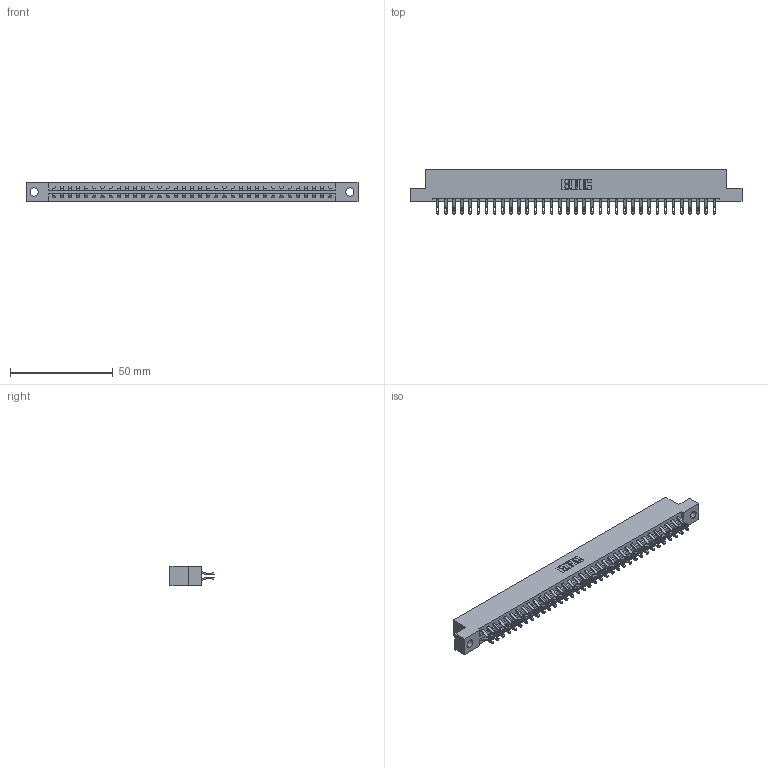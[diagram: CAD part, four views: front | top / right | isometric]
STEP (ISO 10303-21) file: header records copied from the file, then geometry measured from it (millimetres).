
FILE_DESCRIPTION (( 'STEP AP203' ), '1' );
FILE_NAME ('387-070-555-204.STEP', '2019-10-21T22:49:55', ( '' ), ( '' ), 'SwSTEP 2.0', 'SolidWorks 2016', '' );
FILE_SCHEMA (( 'CONFIG_CONTROL_DESIGN' ));
Length unit declared in the file: inch
Products named in the file (3): 345-292-001_555 Tail; 387-070-555-204; 337 Part_Flush Mounting Lugs - 0.156 Dia-TH
Assembly tree (71 placements, depth 2):
  387-070-555-204
    337 Part_Flush Mounting Lugs - 0.156 Dia-TH
    345-292-001_555 Tail  x70
Bounding box: 161.7 x 21.47 x 9.4 mm (x, y, z)
Volume: 17062.9 mm3; surface area: 19784.1 mm2
Topology: 71 solids, 71 shells, 4314 faces, 13541 edges, 9026 vertices
Faces by surface type: plane 2590, cylinder 1724
Entity records: 28371 total; most frequent: CARTESIAN_POINT 4820, ORIENTED_EDGE 4726, DIRECTION 4083, EDGE_CURVE 2363, VECTOR 2215, LINE 2215, VERTEX_POINT 1574, AXIS2_PLACEMENT_3D 934
